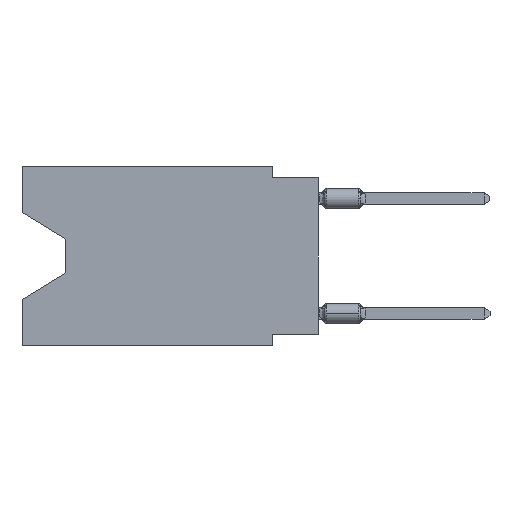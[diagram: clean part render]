
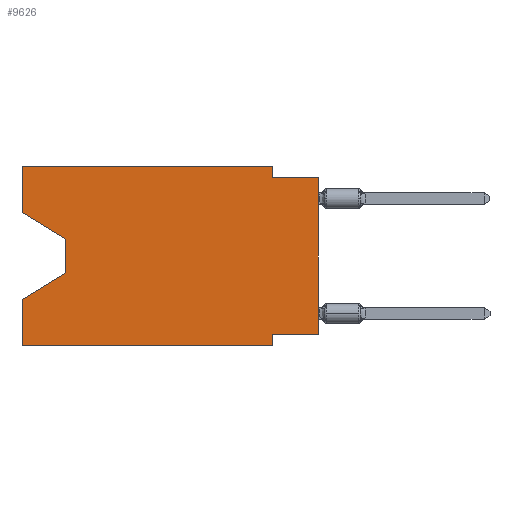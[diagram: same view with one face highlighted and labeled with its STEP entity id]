
A CAD part, left-side view. The second image highlights one B-rep face of the part: STEP entity #9626.
In plain terms, the highlighted planar face has unit normal (-1, 0, 0).
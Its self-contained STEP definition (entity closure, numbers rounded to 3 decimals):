
#104 = VERTEX_POINT ( 'NONE', #4094 ) ;
#503 = VECTOR ( 'NONE', #2105, 1000. ) ;
#817 = DIRECTION ( 'NONE',  ( 0., 0.855, -0.519 ) ) ;
#1078 = VERTEX_POINT ( 'NONE', #19987 ) ;
#1670 = EDGE_CURVE ( 'NONE', #10679, #11632, #13702, .T. ) ;
#2073 = VERTEX_POINT ( 'NONE', #11341 ) ;
#2105 = DIRECTION ( 'NONE',  ( 0., 0., -1. ) ) ;
#2269 = EDGE_CURVE ( 'NONE', #4031, #9731, #2732, .T. ) ;
#2303 = LINE ( 'NONE', #13441, #14054 ) ;
#2323 = EDGE_CURVE ( 'NONE', #11632, #2073, #7490, .T. ) ;
#2380 = VECTOR ( 'NONE', #10941, 1000. ) ;
#2534 = DIRECTION ( 'NONE',  ( 0., -1., 0. ) ) ;
#2732 = LINE ( 'NONE', #17896, #7933 ) ;
#3029 = ORIENTED_EDGE ( 'NONE', *, *, #10922, .T. ) ;
#3162 = CARTESIAN_POINT ( 'NONE',  ( 0., 16.383, -7.36 ) ) ;
#3177 = CARTESIAN_POINT ( 'NONE',  ( 0., 0., -9.271 ) ) ;
#3418 = EDGE_CURVE ( 'NONE', #13247, #2073, #5559, .T. ) ;
#3605 = VECTOR ( 'NONE', #817, 1000. ) ;
#3756 = AXIS2_PLACEMENT_3D ( 'NONE', #10972, #17024, #4780 ) ;
#3860 = EDGE_CURVE ( 'NONE', #13247, #10770, #2303, .T. ) ;
#4031 = VERTEX_POINT ( 'NONE', #16859 ) ;
#4066 = VECTOR ( 'NONE', #19801, 1000. ) ;
#4094 = CARTESIAN_POINT ( 'NONE',  ( 0., 13.97, -4.013 ) ) ;
#4437 = EDGE_CURVE ( 'NONE', #16971, #104, #4674, .T. ) ;
#4608 = EDGE_CURVE ( 'NONE', #15565, #4031, #14540, .T. ) ;
#4651 = VECTOR ( 'NONE', #19856, 1000. ) ;
#4674 = LINE ( 'NONE', #17021, #4066 ) ;
#4780 = DIRECTION ( 'NONE',  ( 0., 0., -1. ) ) ;
#5445 = LINE ( 'NONE', #15074, #14939 ) ;
#5559 = LINE ( 'NONE', #16580, #13724 ) ;
#7042 = EDGE_LOOP ( 'NONE', ( #13351, #9760, #3029, #9110, #19719, #7133, #16944, #14629, #7416, #7993, #8946, #10564 ) ) ;
#7133 = ORIENTED_EDGE ( 'NONE', *, *, #2323, .F. ) ;
#7401 = EDGE_CURVE ( 'NONE', #10679, #9731, #14525, .T. ) ;
#7416 = ORIENTED_EDGE ( 'NONE', *, *, #2269, .F. ) ;
#7490 = LINE ( 'NONE', #9029, #2380 ) ;
#7566 = EDGE_CURVE ( 'NONE', #16597, #15565, #18058, .T. ) ;
#7933 = VECTOR ( 'NONE', #8717, 1000. ) ;
#7993 = ORIENTED_EDGE ( 'NONE', *, *, #4608, .F. ) ;
#8012 = CARTESIAN_POINT ( 'NONE',  ( 0., 16.383, 0. ) ) ;
#8045 = CARTESIAN_POINT ( 'NONE',  ( 0., 2.54, 0. ) ) ;
#8057 = CARTESIAN_POINT ( 'NONE',  ( 0., 16.383, -9.906 ) ) ;
#8330 = CARTESIAN_POINT ( 'NONE',  ( 0., 0., -0.635 ) ) ;
#8491 = DIRECTION ( 'NONE',  ( 0., 0., -1. ) ) ;
#8717 = DIRECTION ( 'NONE',  ( 0., -1., 0. ) ) ;
#8946 = ORIENTED_EDGE ( 'NONE', *, *, #7566, .F. ) ;
#9029 = CARTESIAN_POINT ( 'NONE',  ( 0., 2.54, -9.906 ) ) ;
#9110 = ORIENTED_EDGE ( 'NONE', *, *, #3860, .F. ) ;
#9261 = FACE_OUTER_BOUND ( 'NONE', #7042, .T. ) ;
#9626 = ADVANCED_FACE ( 'NONE', ( #9261 ), #10877, .F. ) ;
#9658 = CARTESIAN_POINT ( 'NONE',  ( 0., 13.97, -5.893 ) ) ;
#9731 = VERTEX_POINT ( 'NONE', #8330 ) ;
#9760 = ORIENTED_EDGE ( 'NONE', *, *, #11382, .T. ) ;
#10317 = DIRECTION ( 'NONE',  ( 0., 0., 1. ) ) ;
#10564 = ORIENTED_EDGE ( 'NONE', *, *, #13492, .F. ) ;
#10679 = VERTEX_POINT ( 'NONE', #18234 ) ;
#10770 = VERTEX_POINT ( 'NONE', #3162 ) ;
#10877 = PLANE ( 'NONE',  #3756 ) ;
#10922 = EDGE_CURVE ( 'NONE', #1078, #10770, #16181, .T. ) ;
#10941 = DIRECTION ( 'NONE',  ( 0., 0., -1. ) ) ;
#10972 = CARTESIAN_POINT ( 'NONE',  ( 0., 16.383, 0. ) ) ;
#11341 = CARTESIAN_POINT ( 'NONE',  ( 0., 2.54, -9.906 ) ) ;
#11382 = EDGE_CURVE ( 'NONE', #104, #1078, #5445, .T. ) ;
#11632 = VERTEX_POINT ( 'NONE', #15735 ) ;
#11769 = VECTOR ( 'NONE', #17655, 1000. ) ;
#11940 = VECTOR ( 'NONE', #18714, 1000. ) ;
#12793 = CARTESIAN_POINT ( 'NONE',  ( 0., 16.383, -2.546 ) ) ;
#13247 = VERTEX_POINT ( 'NONE', #8057 ) ;
#13351 = ORIENTED_EDGE ( 'NONE', *, *, #4437, .T. ) ;
#13441 = CARTESIAN_POINT ( 'NONE',  ( 0., 16.383, 0. ) ) ;
#13492 = EDGE_CURVE ( 'NONE', #16971, #16597, #13953, .T. ) ;
#13702 = LINE ( 'NONE', #3177, #4651 ) ;
#13724 = VECTOR ( 'NONE', #2534, 1000. ) ;
#13953 = LINE ( 'NONE', #8012, #11940 ) ;
#14054 = VECTOR ( 'NONE', #10317, 1000. ) ;
#14342 = CARTESIAN_POINT ( 'NONE',  ( 0., 2.54, 0. ) ) ;
#14525 = LINE ( 'NONE', #19064, #11769 ) ;
#14540 = LINE ( 'NONE', #14342, #503 ) ;
#14629 = ORIENTED_EDGE ( 'NONE', *, *, #7401, .T. ) ;
#14939 = VECTOR ( 'NONE', #8491, 1000. ) ;
#15034 = DIRECTION ( 'NONE',  ( 0., -1., 0. ) ) ;
#15074 = CARTESIAN_POINT ( 'NONE',  ( 0., 13.97, -4.013 ) ) ;
#15139 = CARTESIAN_POINT ( 'NONE',  ( 0., 16.383, 0. ) ) ;
#15565 = VERTEX_POINT ( 'NONE', #8045 ) ;
#15735 = CARTESIAN_POINT ( 'NONE',  ( 0., 2.54, -9.271 ) ) ;
#16181 = LINE ( 'NONE', #9658, #3605 ) ;
#16532 = CARTESIAN_POINT ( 'NONE',  ( 0., 16.383, 0. ) ) ;
#16580 = CARTESIAN_POINT ( 'NONE',  ( 0., 16.383, -9.906 ) ) ;
#16597 = VERTEX_POINT ( 'NONE', #16532 ) ;
#16859 = CARTESIAN_POINT ( 'NONE',  ( 0., 2.54, -0.635 ) ) ;
#16944 = ORIENTED_EDGE ( 'NONE', *, *, #1670, .F. ) ;
#16971 = VERTEX_POINT ( 'NONE', #12793 ) ;
#17021 = CARTESIAN_POINT ( 'NONE',  ( 0., 16.383, -2.546 ) ) ;
#17024 = DIRECTION ( 'NONE',  ( 1., 0., 0. ) ) ;
#17655 = DIRECTION ( 'NONE',  ( 0., 0., 1. ) ) ;
#17896 = CARTESIAN_POINT ( 'NONE',  ( 0., 0., -0.635 ) ) ;
#18058 = LINE ( 'NONE', #15139, #19191 ) ;
#18234 = CARTESIAN_POINT ( 'NONE',  ( 0., 0., -9.271 ) ) ;
#18714 = DIRECTION ( 'NONE',  ( 0., 0., 1. ) ) ;
#19064 = CARTESIAN_POINT ( 'NONE',  ( 0., 0., 0. ) ) ;
#19191 = VECTOR ( 'NONE', #15034, 1000. ) ;
#19719 = ORIENTED_EDGE ( 'NONE', *, *, #3418, .T. ) ;
#19801 = DIRECTION ( 'NONE',  ( 0., -0.855, -0.519 ) ) ;
#19856 = DIRECTION ( 'NONE',  ( 0., 1., 0. ) ) ;
#19987 = CARTESIAN_POINT ( 'NONE',  ( 0., 13.97, -5.893 ) ) ;
